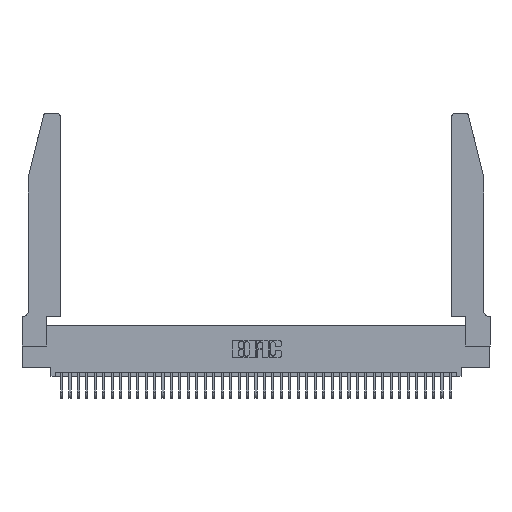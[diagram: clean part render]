
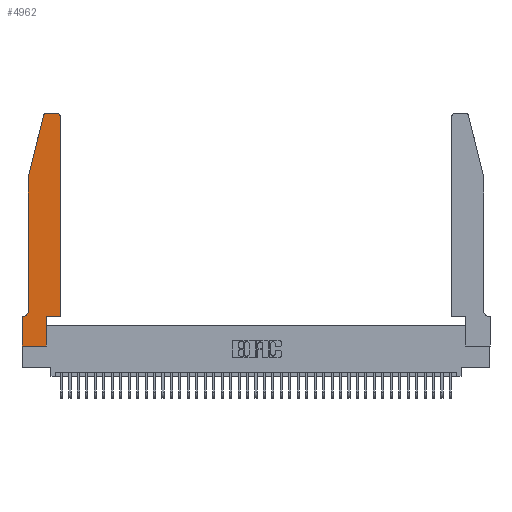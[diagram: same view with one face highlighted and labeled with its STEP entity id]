
A CAD part, top view. The second image highlights one B-rep face of the part: STEP entity #4962.
In plain terms, the highlighted planar face has unit normal (0, 0, 1).
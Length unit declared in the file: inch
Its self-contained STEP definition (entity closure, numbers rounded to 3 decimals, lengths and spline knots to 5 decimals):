
#237 = VERTEX_POINT ( 'NONE', #14484 ) ;
#265 = CARTESIAN_POINT ( 'NONE',  ( 0.25487, 2.72718, 0.37 ) ) ;
#2031 = ORIENTED_EDGE ( 'NONE', *, *, #40225, .T. ) ;
#2870 = VECTOR ( 'NONE', #20203, 39.37008 ) ;
#4417 = EDGE_CURVE ( 'NONE', #42136, #40199, #23478, .T. ) ;
#4433 = DIRECTION ( 'NONE',  ( 0., -1., 0. ) ) ;
#4705 = CARTESIAN_POINT ( 'NONE',  ( 0.2865, 0., 0.37 ) ) ;
#4962 = ADVANCED_FACE ( 'NONE', ( #39885 ), #11228, .T. ) ;
#4993 = EDGE_CURVE ( 'NONE', #19942, #15582, #10558, .T. ) ;
#6370 = DIRECTION ( 'NONE',  ( 1., 0., 0. ) ) ;
#6402 = CARTESIAN_POINT ( 'NONE',  ( 0.4205, 2.75, 0.37 ) ) ;
#7518 = ORIENTED_EDGE ( 'NONE', *, *, #7896, .T. ) ;
#7896 = EDGE_CURVE ( 'NONE', #35202, #11003, #31202, .T. ) ;
#8675 = EDGE_CURVE ( 'NONE', #15623, #41702, #14142, .T. ) ;
#8834 = DIRECTION ( 'NONE',  ( 0., 0., 1. ) ) ;
#9034 = LINE ( 'NONE', #24275, #18841 ) ;
#9566 = DIRECTION ( 'NONE',  ( 0., -1., 0. ) ) ;
#10016 = CARTESIAN_POINT ( 'NONE',  ( 0.0755, 0.42, 0.37 ) ) ;
#10060 = ORIENTED_EDGE ( 'NONE', *, *, #32126, .T. ) ;
#10558 = CIRCLE ( 'NONE', #18727, 0.07 ) ;
#10742 = VERTEX_POINT ( 'NONE', #18341 ) ;
#11003 = VERTEX_POINT ( 'NONE', #6402 ) ;
#11228 = PLANE ( 'NONE',  #20927 ) ;
#11371 = DIRECTION ( 'NONE',  ( 0., 0., -1. ) ) ;
#11778 = LINE ( 'NONE', #13582, #2870 ) ;
#12827 = EDGE_LOOP ( 'NONE', ( #34499, #33638, #25992, #22522, #36557, #29435, #10060, #22928, #37579, #2031, #37804, #7518 ) ) ;
#13097 = VECTOR ( 'NONE', #6370, 39.37008 ) ;
#13133 = CARTESIAN_POINT ( 'NONE',  ( 0.0755, 0.35, 0.37 ) ) ;
#13570 = CARTESIAN_POINT ( 'NONE',  ( 0.284, 2.75, 0.37 ) ) ;
#13582 = CARTESIAN_POINT ( 'NONE',  ( 0.2865, 0.35, 0.37 ) ) ;
#13938 = CARTESIAN_POINT ( 'NONE',  ( 0.4505, 0.35, 0.37 ) ) ;
#13987 = DIRECTION ( 'NONE',  ( 0., 0., 1. ) ) ;
#14124 = LINE ( 'NONE', #13938, #30614 ) ;
#14142 = LINE ( 'NONE', #19707, #13097 ) ;
#14331 = DIRECTION ( 'NONE',  ( 0., 1., 0. ) ) ;
#14484 = CARTESIAN_POINT ( 'NONE',  ( 0.2865, 0.35, 0.37 ) ) ;
#14537 = DIRECTION ( 'NONE',  ( 1., 0., 0. ) ) ;
#14711 = EDGE_CURVE ( 'NONE', #40199, #19942, #33777, .T. ) ;
#15034 = VECTOR ( 'NONE', #16612, 39.37008 ) ;
#15440 = VERTEX_POINT ( 'NONE', #13570 ) ;
#15493 = CIRCLE ( 'NONE', #28164, 0.03 ) ;
#15582 = VERTEX_POINT ( 'NONE', #34150 ) ;
#15623 = VERTEX_POINT ( 'NONE', #17900 ) ;
#15925 = VECTOR ( 'NONE', #14331, 39.37008 ) ;
#16612 = DIRECTION ( 'NONE',  ( -1., 0., 0. ) ) ;
#17374 = LINE ( 'NONE', #27221, #33842 ) ;
#17599 = CARTESIAN_POINT ( 'NONE',  ( 0.0755, 2., 0.37 ) ) ;
#17900 = CARTESIAN_POINT ( 'NONE',  ( 0., 0., 0.37 ) ) ;
#18341 = CARTESIAN_POINT ( 'NONE',  ( 0.4505, 0.35, 0.37 ) ) ;
#18727 = AXIS2_PLACEMENT_3D ( 'NONE', #31070, #11371, #34396 ) ;
#18841 = VECTOR ( 'NONE', #4433, 39.37008 ) ;
#18853 = EDGE_CURVE ( 'NONE', #41702, #237, #11778, .T. ) ;
#19707 = CARTESIAN_POINT ( 'NONE',  ( 0., 0., 0.37 ) ) ;
#19942 = VERTEX_POINT ( 'NONE', #10016 ) ;
#20203 = DIRECTION ( 'NONE',  ( 0., 1., 0. ) ) ;
#20406 = CARTESIAN_POINT ( 'NONE',  ( 0.0755, 2., 0.37 ) ) ;
#20927 = AXIS2_PLACEMENT_3D ( 'NONE', #24330, #34257, #14537 ) ;
#21466 = VERTEX_POINT ( 'NONE', #35216 ) ;
#21876 = EDGE_CURVE ( 'NONE', #10742, #35202, #42114, .T. ) ;
#21912 = VECTOR ( 'NONE', #9566, 39.37008 ) ;
#22522 = ORIENTED_EDGE ( 'NONE', *, *, #14711, .T. ) ;
#22928 = ORIENTED_EDGE ( 'NONE', *, *, #8675, .T. ) ;
#23017 = EDGE_CURVE ( 'NONE', #11003, #15440, #17374, .T. ) ;
#23478 = LINE ( 'NONE', #17599, #31205 ) ;
#23772 = LINE ( 'NONE', #13133, #15034 ) ;
#24210 = DIRECTION ( 'NONE',  ( -0.239, -0.971, 0. ) ) ;
#24275 = CARTESIAN_POINT ( 'NONE',  ( 0., 0., 0.37 ) ) ;
#24330 = CARTESIAN_POINT ( 'NONE',  ( 0., 0.35, 0.37 ) ) ;
#25418 = AXIS2_PLACEMENT_3D ( 'NONE', #28592, #8834, #31868 ) ;
#25992 = ORIENTED_EDGE ( 'NONE', *, *, #4417, .T. ) ;
#26730 = EDGE_CURVE ( 'NONE', #15582, #21466, #23772, .T. ) ;
#27221 = CARTESIAN_POINT ( 'NONE',  ( 0.2605, 2.75, 0.37 ) ) ;
#27886 = CARTESIAN_POINT ( 'NONE',  ( 0.4505, 2.72, 0.37 ) ) ;
#28164 = AXIS2_PLACEMENT_3D ( 'NONE', #33702, #13987, #37015 ) ;
#28592 = CARTESIAN_POINT ( 'NONE',  ( 0.4205, 2.72, 0.37 ) ) ;
#28769 = EDGE_CURVE ( 'NONE', #15440, #42136, #15493, .T. ) ;
#29435 = ORIENTED_EDGE ( 'NONE', *, *, #26730, .T. ) ;
#30614 = VECTOR ( 'NONE', #40096, 39.37008 ) ;
#30736 = CARTESIAN_POINT ( 'NONE',  ( 0.4505, 0.35, 0.37 ) ) ;
#31070 = CARTESIAN_POINT ( 'NONE',  ( 0.0055, 0.42, 0.37 ) ) ;
#31202 = CIRCLE ( 'NONE', #25418, 0.03 ) ;
#31205 = VECTOR ( 'NONE', #24210, 39.37008 ) ;
#31868 = DIRECTION ( 'NONE',  ( 1., 0., 0. ) ) ;
#32126 = EDGE_CURVE ( 'NONE', #21466, #15623, #9034, .T. ) ;
#32594 = CARTESIAN_POINT ( 'NONE',  ( 0.0755, 2., 0.37 ) ) ;
#33638 = ORIENTED_EDGE ( 'NONE', *, *, #28769, .T. ) ;
#33702 = CARTESIAN_POINT ( 'NONE',  ( 0.284, 2.72, 0.37 ) ) ;
#33777 = LINE ( 'NONE', #32594, #21912 ) ;
#33842 = VECTOR ( 'NONE', #40404, 39.37008 ) ;
#34150 = CARTESIAN_POINT ( 'NONE',  ( 0.0055, 0.35, 0.37 ) ) ;
#34257 = DIRECTION ( 'NONE',  ( 0., 0., 1. ) ) ;
#34396 = DIRECTION ( 'NONE',  ( -1., 0., 0. ) ) ;
#34499 = ORIENTED_EDGE ( 'NONE', *, *, #23017, .T. ) ;
#35202 = VERTEX_POINT ( 'NONE', #27886 ) ;
#35216 = CARTESIAN_POINT ( 'NONE',  ( 0., 0.35, 0.37 ) ) ;
#36557 = ORIENTED_EDGE ( 'NONE', *, *, #4993, .T. ) ;
#37015 = DIRECTION ( 'NONE',  ( 1., 0., 0. ) ) ;
#37579 = ORIENTED_EDGE ( 'NONE', *, *, #18853, .T. ) ;
#37804 = ORIENTED_EDGE ( 'NONE', *, *, #21876, .T. ) ;
#39885 = FACE_OUTER_BOUND ( 'NONE', #12827, .T. ) ;
#40096 = DIRECTION ( 'NONE',  ( 1., 0., 0. ) ) ;
#40199 = VERTEX_POINT ( 'NONE', #20406 ) ;
#40225 = EDGE_CURVE ( 'NONE', #237, #10742, #14124, .T. ) ;
#40404 = DIRECTION ( 'NONE',  ( -1., 0., 0. ) ) ;
#41702 = VERTEX_POINT ( 'NONE', #4705 ) ;
#42114 = LINE ( 'NONE', #30736, #15925 ) ;
#42136 = VERTEX_POINT ( 'NONE', #265 ) ;
